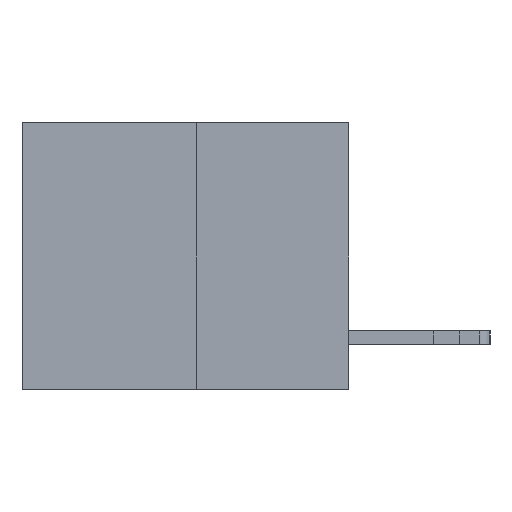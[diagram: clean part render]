
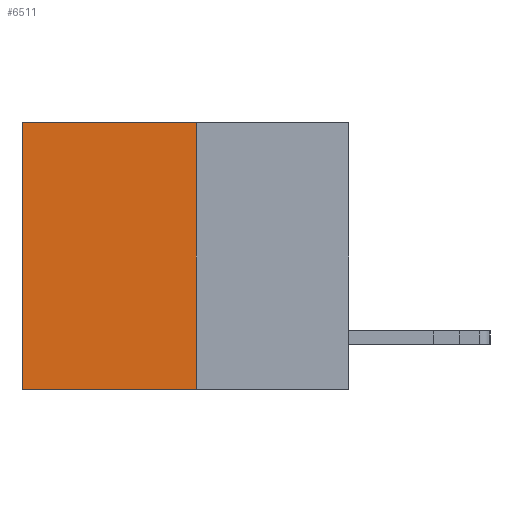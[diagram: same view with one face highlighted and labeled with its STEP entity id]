
A CAD part, left-side view. The second image highlights one B-rep face of the part: STEP entity #6511.
In plain terms, the highlighted planar face has unit normal (-1, 0, 0).
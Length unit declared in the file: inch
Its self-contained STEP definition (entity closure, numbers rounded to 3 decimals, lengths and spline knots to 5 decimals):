
#523 = ORIENTED_EDGE ( 'NONE', *, *, #10871, .T. ) ;
#607 = CARTESIAN_POINT ( 'NONE',  ( 0.3165, 0.6, 0. ) ) ;
#2016 = EDGE_CURVE ( 'NONE', #18005, #8775, #13251, .T. ) ;
#2161 = LINE ( 'NONE', #3197, #14843 ) ;
#2510 = DIRECTION ( 'NONE',  ( 1., 0., 0. ) ) ;
#3197 = CARTESIAN_POINT ( 'NONE',  ( 0.3165, 0.6, -0.49 ) ) ;
#4400 = ORIENTED_EDGE ( 'NONE', *, *, #2016, .F. ) ;
#4692 = VERTEX_POINT ( 'NONE', #607 ) ;
#4915 = CARTESIAN_POINT ( 'NONE',  ( 0.3165, 0.28, -0.49 ) ) ;
#5169 = LINE ( 'NONE', #4915, #18110 ) ;
#5479 = EDGE_LOOP ( 'NONE', ( #16120, #4400, #23226, #523 ) ) ;
#6511 = ADVANCED_FACE ( 'NONE', ( #22492 ), #17557, .F. ) ;
#6572 = CARTESIAN_POINT ( 'NONE',  ( 0.3165, 0.28, 0. ) ) ;
#6992 = CARTESIAN_POINT ( 'NONE',  ( 0.3165, 0.28, -0.49 ) ) ;
#8553 = CARTESIAN_POINT ( 'NONE',  ( 0.3165, 0.28, 0. ) ) ;
#8638 = DIRECTION ( 'NONE',  ( 0., 1., 0. ) ) ;
#8775 = VERTEX_POINT ( 'NONE', #13277 ) ;
#9123 = CARTESIAN_POINT ( 'NONE',  ( 0.3165, 0.28, -0.49 ) ) ;
#10871 = EDGE_CURVE ( 'NONE', #15286, #4692, #22246, .T. ) ;
#12474 = AXIS2_PLACEMENT_3D ( 'NONE', #9123, #2510, #23961 ) ;
#13251 = LINE ( 'NONE', #6992, #16572 ) ;
#13277 = CARTESIAN_POINT ( 'NONE',  ( 0.3165, 0.6, -0.49 ) ) ;
#13970 = DIRECTION ( 'NONE',  ( 0., 0., -1. ) ) ;
#14843 = VECTOR ( 'NONE', #13970, 39.37008 ) ;
#15286 = VERTEX_POINT ( 'NONE', #6572 ) ;
#16120 = ORIENTED_EDGE ( 'NONE', *, *, #16859, .T. ) ;
#16572 = VECTOR ( 'NONE', #21859, 39.37008 ) ;
#16859 = EDGE_CURVE ( 'NONE', #4692, #8775, #2161, .T. ) ;
#17305 = EDGE_CURVE ( 'NONE', #15286, #18005, #5169, .T. ) ;
#17557 = PLANE ( 'NONE',  #12474 ) ;
#18005 = VERTEX_POINT ( 'NONE', #20784 ) ;
#18110 = VECTOR ( 'NONE', #26008, 39.37008 ) ;
#20784 = CARTESIAN_POINT ( 'NONE',  ( 0.3165, 0.28, -0.49 ) ) ;
#21572 = VECTOR ( 'NONE', #8638, 39.37008 ) ;
#21859 = DIRECTION ( 'NONE',  ( 0., 1., 0. ) ) ;
#22246 = LINE ( 'NONE', #8553, #21572 ) ;
#22492 = FACE_OUTER_BOUND ( 'NONE', #5479, .T. ) ;
#23226 = ORIENTED_EDGE ( 'NONE', *, *, #17305, .F. ) ;
#23961 = DIRECTION ( 'NONE',  ( 0., 0., -1. ) ) ;
#26008 = DIRECTION ( 'NONE',  ( 0., 0., -1. ) ) ;
